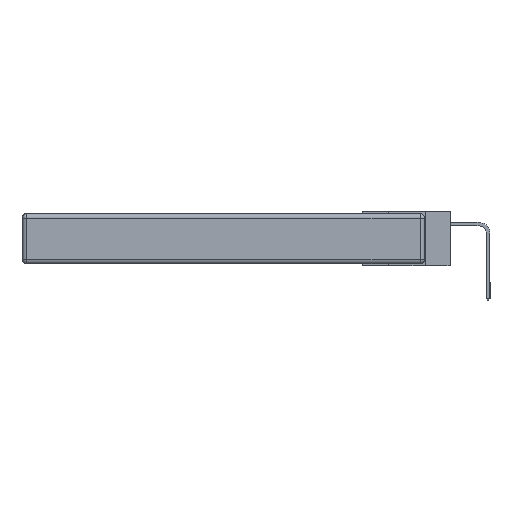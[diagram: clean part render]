
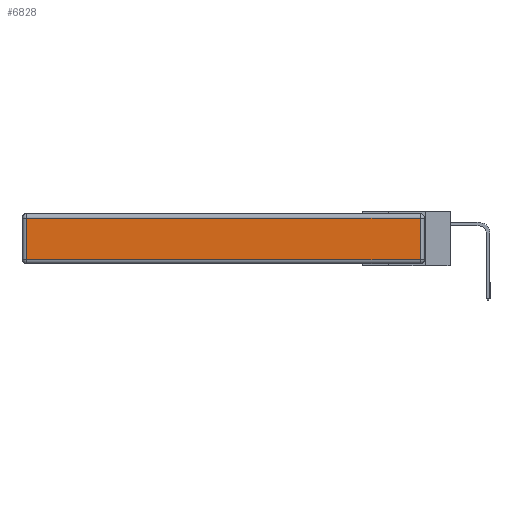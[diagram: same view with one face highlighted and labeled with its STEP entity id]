
A CAD part, left-side view. The second image highlights one B-rep face of the part: STEP entity #6828.
In plain terms, the highlighted planar face has unit normal (-1, 0, 0).
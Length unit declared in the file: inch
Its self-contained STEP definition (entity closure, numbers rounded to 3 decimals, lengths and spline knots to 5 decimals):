
#482 = ORIENTED_EDGE ( 'NONE', *, *, #24066, .T. ) ;
#2310 = VECTOR ( 'NONE', #27935, 39.37008 ) ;
#2352 = VERTEX_POINT ( 'NONE', #19157 ) ;
#4493 = AXIS2_PLACEMENT_3D ( 'NONE', #26224, #23379, #25896 ) ;
#6324 = CARTESIAN_POINT ( 'NONE',  ( 0., 0.03, -0.03 ) ) ;
#6828 = ADVANCED_FACE ( 'NONE', ( #30650 ), #7427, .T. ) ;
#7427 = PLANE ( 'NONE',  #4493 ) ;
#7662 = DIRECTION ( 'NONE',  ( 0., 0., -1. ) ) ;
#10817 = LINE ( 'NONE', #27535, #17040 ) ;
#10929 = VERTEX_POINT ( 'NONE', #6324 ) ;
#13398 = EDGE_CURVE ( 'NONE', #2352, #18832, #22044, .T. ) ;
#13462 = LINE ( 'NONE', #30952, #2310 ) ;
#14165 = CARTESIAN_POINT ( 'NONE',  ( 0., 0.03, -0.313 ) ) ;
#15342 = VECTOR ( 'NONE', #23863, 39.37008 ) ;
#17040 = VECTOR ( 'NONE', #17193, 39.37008 ) ;
#17193 = DIRECTION ( 'NONE',  ( 0., 1., 0. ) ) ;
#17818 = CARTESIAN_POINT ( 'NONE',  ( 0., 2.72, -0.313 ) ) ;
#17914 = VECTOR ( 'NONE', #7662, 39.37008 ) ;
#18832 = VERTEX_POINT ( 'NONE', #17818 ) ;
#19157 = CARTESIAN_POINT ( 'NONE',  ( 0., 2.72, -0.03 ) ) ;
#20723 = LINE ( 'NONE', #29033, #15342 ) ;
#21128 = EDGE_CURVE ( 'NONE', #10929, #2352, #10817, .T. ) ;
#21146 = ORIENTED_EDGE ( 'NONE', *, *, #13398, .T. ) ;
#22044 = LINE ( 'NONE', #25912, #17914 ) ;
#22240 = VERTEX_POINT ( 'NONE', #14165 ) ;
#23379 = DIRECTION ( 'NONE',  ( -1., 0., 0. ) ) ;
#23863 = DIRECTION ( 'NONE',  ( 0., -1., 0. ) ) ;
#24066 = EDGE_CURVE ( 'NONE', #18832, #22240, #20723, .T. ) ;
#24614 = EDGE_LOOP ( 'NONE', ( #482, #27909, #33106, #21146 ) ) ;
#25896 = DIRECTION ( 'NONE',  ( 0., 0., 1. ) ) ;
#25912 = CARTESIAN_POINT ( 'NONE',  ( 0., 2.72, -0.343 ) ) ;
#26224 = CARTESIAN_POINT ( 'NONE',  ( 0., 0., -0.343 ) ) ;
#27535 = CARTESIAN_POINT ( 'NONE',  ( 0., 2.75, -0.03 ) ) ;
#27909 = ORIENTED_EDGE ( 'NONE', *, *, #33412, .T. ) ;
#27935 = DIRECTION ( 'NONE',  ( 0., 0., 1. ) ) ;
#29033 = CARTESIAN_POINT ( 'NONE',  ( 0., 0., -0.313 ) ) ;
#30650 = FACE_OUTER_BOUND ( 'NONE', #24614, .T. ) ;
#30952 = CARTESIAN_POINT ( 'NONE',  ( 0., 0.03, -0.343 ) ) ;
#33106 = ORIENTED_EDGE ( 'NONE', *, *, #21128, .T. ) ;
#33412 = EDGE_CURVE ( 'NONE', #22240, #10929, #13462, .T. ) ;
